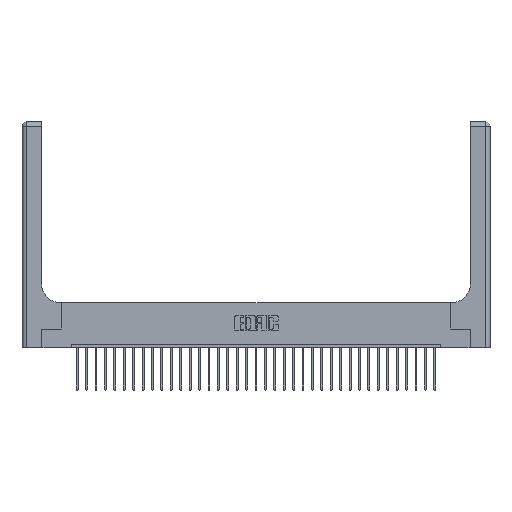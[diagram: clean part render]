
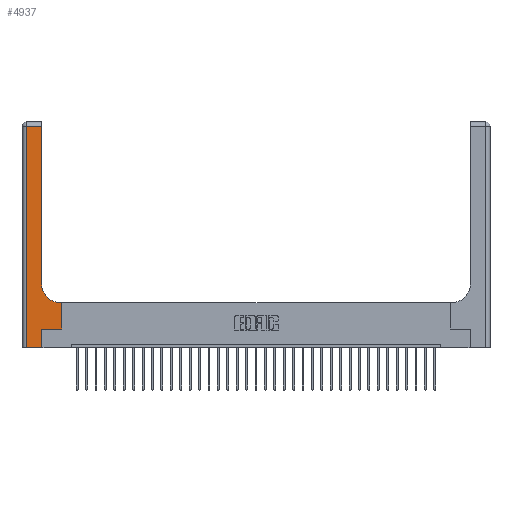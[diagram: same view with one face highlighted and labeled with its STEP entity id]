
A CAD part, top view. The second image highlights one B-rep face of the part: STEP entity #4937.
In plain terms, the highlighted planar face has unit normal (0, 0, 1).
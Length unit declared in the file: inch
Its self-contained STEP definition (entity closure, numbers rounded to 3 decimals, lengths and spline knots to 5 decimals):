
#843 = CARTESIAN_POINT ( 'NONE',  ( 0.26, 2.94, 0.37 ) ) ;
#895 = VERTEX_POINT ( 'NONE', #22274 ) ;
#1322 = VERTEX_POINT ( 'NONE', #843 ) ;
#1667 = DIRECTION ( 'NONE',  ( 1., 0., 0. ) ) ;
#1676 = CARTESIAN_POINT ( 'NONE',  ( 0.528, 0.25, 0.37 ) ) ;
#1816 = CARTESIAN_POINT ( 'NONE',  ( 0.51, 0.85, 0.37 ) ) ;
#3922 = VERTEX_POINT ( 'NONE', #26464 ) ;
#4147 = DIRECTION ( 'NONE',  ( 1., 0., 0. ) ) ;
#4222 = VERTEX_POINT ( 'NONE', #20147 ) ;
#4430 = LINE ( 'NONE', #13287, #19145 ) ;
#4826 = DIRECTION ( 'NONE',  ( -1., 0., 0. ) ) ;
#4937 = ADVANCED_FACE ( 'NONE', ( #20428 ), #21394, .F. ) ;
#5312 = ORIENTED_EDGE ( 'NONE', *, *, #17266, .T. ) ;
#5401 = CARTESIAN_POINT ( 'NONE',  ( 0., 3., 0.37 ) ) ;
#6351 = EDGE_CURVE ( 'NONE', #895, #19730, #9931, .T. ) ;
#6659 = LINE ( 'NONE', #13475, #21726 ) ;
#7157 = CARTESIAN_POINT ( 'NONE',  ( 0.265, 0., 0.37 ) ) ;
#7475 = LINE ( 'NONE', #1676, #9989 ) ;
#7929 = VERTEX_POINT ( 'NONE', #28324 ) ;
#8212 = ORIENTED_EDGE ( 'NONE', *, *, #17547, .T. ) ;
#8346 = VECTOR ( 'NONE', #15785, 39.37008 ) ;
#8535 = DIRECTION ( 'NONE',  ( 0., 1., 0. ) ) ;
#8541 = DIRECTION ( 'NONE',  ( -1., 0., 0. ) ) ;
#9088 = EDGE_CURVE ( 'NONE', #10538, #1322, #4430, .T. ) ;
#9172 = CARTESIAN_POINT ( 'NONE',  ( 0., 2.94, 0.37 ) ) ;
#9242 = VECTOR ( 'NONE', #18711, 39.37008 ) ;
#9931 = LINE ( 'NONE', #7157, #9242 ) ;
#9989 = VECTOR ( 'NONE', #8535, 39.37008 ) ;
#10045 = DIRECTION ( 'NONE',  ( -1., 0., 0. ) ) ;
#10120 = LINE ( 'NONE', #13895, #8346 ) ;
#10538 = VERTEX_POINT ( 'NONE', #24395 ) ;
#11152 = DIRECTION ( 'NONE',  ( 0., 0., -1. ) ) ;
#11386 = AXIS2_PLACEMENT_3D ( 'NONE', #5401, #23978, #10045 ) ;
#11635 = EDGE_CURVE ( 'NONE', #1322, #17114, #21760, .T. ) ;
#12819 = AXIS2_PLACEMENT_3D ( 'NONE', #1816, #11152, #4147 ) ;
#13208 = LINE ( 'NONE', #29326, #26450 ) ;
#13240 = CARTESIAN_POINT ( 'NONE',  ( 0.51, 0.6, 0.37 ) ) ;
#13287 = CARTESIAN_POINT ( 'NONE',  ( 0.26, 3., 0.37 ) ) ;
#13372 = ORIENTED_EDGE ( 'NONE', *, *, #22473, .T. ) ;
#13475 = CARTESIAN_POINT ( 'NONE',  ( 0.265, 0.25, 0.37 ) ) ;
#13895 = CARTESIAN_POINT ( 'NONE',  ( 0.06, 3., 0.37 ) ) ;
#14417 = VECTOR ( 'NONE', #1667, 39.37008 ) ;
#15556 = EDGE_LOOP ( 'NONE', ( #23290, #20717, #29419, #13372, #24730, #29163, #5312, #8212, #19464 ) ) ;
#15785 = DIRECTION ( 'NONE',  ( 0., -1., 0. ) ) ;
#16354 = EDGE_CURVE ( 'NONE', #20736, #10538, #20467, .T. ) ;
#16902 = LINE ( 'NONE', #22370, #14417 ) ;
#17114 = VERTEX_POINT ( 'NONE', #20306 ) ;
#17266 = EDGE_CURVE ( 'NONE', #4222, #7929, #7475, .T. ) ;
#17547 = EDGE_CURVE ( 'NONE', #7929, #20736, #13208, .T. ) ;
#17983 = CARTESIAN_POINT ( 'NONE',  ( 0.265, 0.25, 0.37 ) ) ;
#18711 = DIRECTION ( 'NONE',  ( 0., 1., 0. ) ) ;
#19145 = VECTOR ( 'NONE', #24614, 39.37008 ) ;
#19464 = ORIENTED_EDGE ( 'NONE', *, *, #16354, .T. ) ;
#19730 = VERTEX_POINT ( 'NONE', #17983 ) ;
#19755 = EDGE_CURVE ( 'NONE', #19730, #4222, #6659, .T. ) ;
#19983 = VECTOR ( 'NONE', #4826, 39.37008 ) ;
#20147 = CARTESIAN_POINT ( 'NONE',  ( 0.528, 0.25, 0.37 ) ) ;
#20306 = CARTESIAN_POINT ( 'NONE',  ( 0.06, 2.94, 0.37 ) ) ;
#20428 = FACE_OUTER_BOUND ( 'NONE', #15556, .T. ) ;
#20467 = CIRCLE ( 'NONE', #12819, 0.25 ) ;
#20717 = ORIENTED_EDGE ( 'NONE', *, *, #11635, .T. ) ;
#20736 = VERTEX_POINT ( 'NONE', #13240 ) ;
#21338 = EDGE_CURVE ( 'NONE', #17114, #3922, #10120, .T. ) ;
#21394 = PLANE ( 'NONE',  #11386 ) ;
#21726 = VECTOR ( 'NONE', #22606, 39.37008 ) ;
#21760 = LINE ( 'NONE', #9172, #19983 ) ;
#22274 = CARTESIAN_POINT ( 'NONE',  ( 0.265, 0., 0.37 ) ) ;
#22370 = CARTESIAN_POINT ( 'NONE',  ( 0., 0., 0.37 ) ) ;
#22473 = EDGE_CURVE ( 'NONE', #3922, #895, #16902, .T. ) ;
#22606 = DIRECTION ( 'NONE',  ( 1., 0., 0. ) ) ;
#23290 = ORIENTED_EDGE ( 'NONE', *, *, #9088, .T. ) ;
#23978 = DIRECTION ( 'NONE',  ( 0., 0., -1. ) ) ;
#24395 = CARTESIAN_POINT ( 'NONE',  ( 0.26, 0.85, 0.37 ) ) ;
#24614 = DIRECTION ( 'NONE',  ( 0., 1., 0. ) ) ;
#24730 = ORIENTED_EDGE ( 'NONE', *, *, #6351, .T. ) ;
#26450 = VECTOR ( 'NONE', #8541, 39.37008 ) ;
#26464 = CARTESIAN_POINT ( 'NONE',  ( 0.06, 0., 0.37 ) ) ;
#28324 = CARTESIAN_POINT ( 'NONE',  ( 0.528, 0.6, 0.37 ) ) ;
#29163 = ORIENTED_EDGE ( 'NONE', *, *, #19755, .T. ) ;
#29326 = CARTESIAN_POINT ( 'NONE',  ( 0.26, 0.6, 0.37 ) ) ;
#29419 = ORIENTED_EDGE ( 'NONE', *, *, #21338, .T. ) ;
